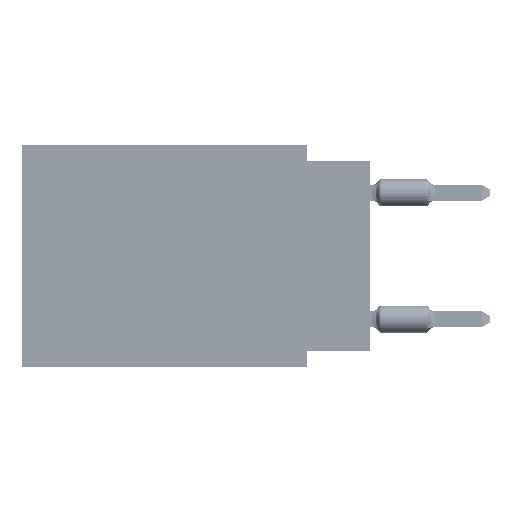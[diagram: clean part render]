
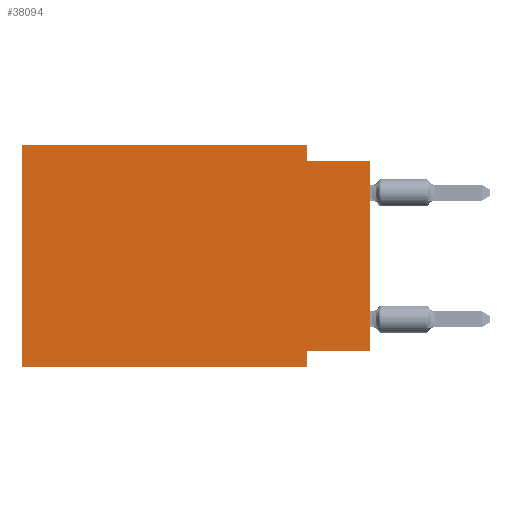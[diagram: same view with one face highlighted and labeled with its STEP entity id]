
A CAD part, left-side view. The second image highlights one B-rep face of the part: STEP entity #38094.
In plain terms, the highlighted planar face has unit normal (-1, 0, 0).
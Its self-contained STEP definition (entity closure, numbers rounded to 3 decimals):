
#3361 = EDGE_CURVE ( 'NONE', #29950, #13207, #57841, .T. ) ;
#4995 = DIRECTION ( 'NONE',  ( 0., 0., 1. ) ) ;
#6256 = CARTESIAN_POINT ( 'NONE',  ( 0., 2.54, -8.255 ) ) ;
#6839 = DIRECTION ( 'NONE',  ( 0., 0., -1. ) ) ;
#8117 = CARTESIAN_POINT ( 'NONE',  ( 0., 13.97, 0. ) ) ;
#9822 = VERTEX_POINT ( 'NONE', #92503 ) ;
#9897 = CARTESIAN_POINT ( 'NONE',  ( 0., 13.97, 0. ) ) ;
#11811 = VERTEX_POINT ( 'NONE', #42435 ) ;
#13207 = VERTEX_POINT ( 'NONE', #99254 ) ;
#15279 = EDGE_CURVE ( 'NONE', #29950, #86218, #88317, .T. ) ;
#23721 = EDGE_LOOP ( 'NONE', ( #31060, #31069, #65783, #95186, #86768, #86665, #45917, #62657 ) ) ;
#24145 = DIRECTION ( 'NONE',  ( 1., 0., 0. ) ) ;
#27563 = VECTOR ( 'NONE', #82837, 1000. ) ;
#27626 = VECTOR ( 'NONE', #90673, 1000. ) ;
#29228 = CARTESIAN_POINT ( 'NONE',  ( 0., 0., -8.255 ) ) ;
#29950 = VERTEX_POINT ( 'NONE', #66211 ) ;
#30191 = VERTEX_POINT ( 'NONE', #6256 ) ;
#31060 = ORIENTED_EDGE ( 'NONE', *, *, #79892, .T. ) ;
#31069 = ORIENTED_EDGE ( 'NONE', *, *, #45591, .F. ) ;
#31142 = VECTOR ( 'NONE', #4995, 1000. ) ;
#32255 = PLANE ( 'NONE',  #79822 ) ;
#33772 = FACE_OUTER_BOUND ( 'NONE', #23721, .T. ) ;
#34957 = VECTOR ( 'NONE', #55832, 1000. ) ;
#37634 = VECTOR ( 'NONE', #6839, 1000. ) ;
#38094 = ADVANCED_FACE ( 'NONE', ( #33772 ), #32255, .F. ) ;
#42435 = CARTESIAN_POINT ( 'NONE',  ( 0., 0., -8.255 ) ) ;
#43587 = CARTESIAN_POINT ( 'NONE',  ( 0., 13.97, 0. ) ) ;
#43865 = VERTEX_POINT ( 'NONE', #72305 ) ;
#45591 = EDGE_CURVE ( 'NONE', #43865, #99969, #56780, .T. ) ;
#45917 = ORIENTED_EDGE ( 'NONE', *, *, #57880, .F. ) ;
#47992 = DIRECTION ( 'NONE',  ( 0., 0., -1. ) ) ;
#48166 = CARTESIAN_POINT ( 'NONE',  ( 0., 0., -0.635 ) ) ;
#51863 = LINE ( 'NONE', #59967, #27563 ) ;
#52938 = DIRECTION ( 'NONE',  ( 0., 0., 1. ) ) ;
#55832 = DIRECTION ( 'NONE',  ( 0., -1., 0. ) ) ;
#56780 = LINE ( 'NONE', #48166, #60046 ) ;
#57832 = DIRECTION ( 'NONE',  ( 0., -1., 0. ) ) ;
#57841 = LINE ( 'NONE', #43587, #31142 ) ;
#57880 = EDGE_CURVE ( 'NONE', #30191, #86218, #91140, .T. ) ;
#58694 = LINE ( 'NONE', #29228, #27626 ) ;
#59967 = CARTESIAN_POINT ( 'NONE',  ( 0., 2.54, 0. ) ) ;
#60046 = VECTOR ( 'NONE', #64892, 1000. ) ;
#60539 = CARTESIAN_POINT ( 'NONE',  ( 0., 0., 0. ) ) ;
#62657 = ORIENTED_EDGE ( 'NONE', *, *, #88849, .F. ) ;
#64892 = DIRECTION ( 'NONE',  ( 0., -1., 0. ) ) ;
#65783 = ORIENTED_EDGE ( 'NONE', *, *, #96910, .F. ) ;
#66211 = CARTESIAN_POINT ( 'NONE',  ( 0., 13.97, -8.89 ) ) ;
#69172 = LINE ( 'NONE', #60539, #74897 ) ;
#70062 = LINE ( 'NONE', #8117, #34957 ) ;
#72305 = CARTESIAN_POINT ( 'NONE',  ( 0., 2.54, -0.635 ) ) ;
#74897 = VECTOR ( 'NONE', #52938, 1000. ) ;
#79614 = VECTOR ( 'NONE', #57832, 1000. ) ;
#79822 = AXIS2_PLACEMENT_3D ( 'NONE', #9897, #24145, #47992 ) ;
#79892 = EDGE_CURVE ( 'NONE', #11811, #99969, #69172, .T. ) ;
#81691 = EDGE_CURVE ( 'NONE', #13207, #9822, #70062, .T. ) ;
#82032 = CARTESIAN_POINT ( 'NONE',  ( 0., 2.54, -8.89 ) ) ;
#82328 = CARTESIAN_POINT ( 'NONE',  ( 0., 0., -0.635 ) ) ;
#82837 = DIRECTION ( 'NONE',  ( 0., 0., -1. ) ) ;
#86218 = VERTEX_POINT ( 'NONE', #86493 ) ;
#86493 = CARTESIAN_POINT ( 'NONE',  ( 0., 2.54, -8.89 ) ) ;
#86665 = ORIENTED_EDGE ( 'NONE', *, *, #15279, .T. ) ;
#86768 = ORIENTED_EDGE ( 'NONE', *, *, #3361, .F. ) ;
#88317 = LINE ( 'NONE', #89800, #79614 ) ;
#88849 = EDGE_CURVE ( 'NONE', #11811, #30191, #58694, .T. ) ;
#89800 = CARTESIAN_POINT ( 'NONE',  ( 0., 13.97, -8.89 ) ) ;
#90673 = DIRECTION ( 'NONE',  ( 0., 1., 0. ) ) ;
#91140 = LINE ( 'NONE', #82032, #37634 ) ;
#92503 = CARTESIAN_POINT ( 'NONE',  ( 0., 2.54, 0. ) ) ;
#95186 = ORIENTED_EDGE ( 'NONE', *, *, #81691, .F. ) ;
#96910 = EDGE_CURVE ( 'NONE', #9822, #43865, #51863, .T. ) ;
#99254 = CARTESIAN_POINT ( 'NONE',  ( 0., 13.97, 0. ) ) ;
#99969 = VERTEX_POINT ( 'NONE', #82328 ) ;
